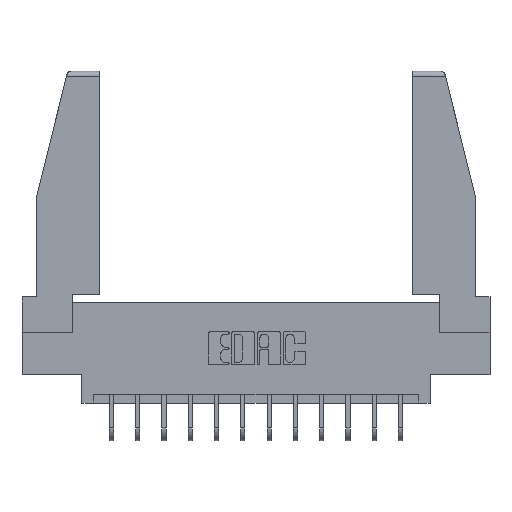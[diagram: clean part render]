
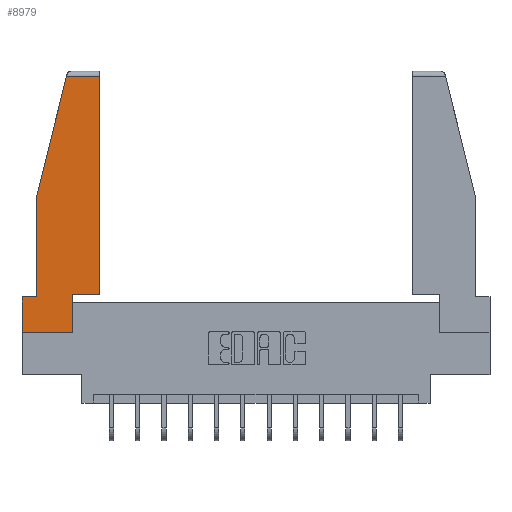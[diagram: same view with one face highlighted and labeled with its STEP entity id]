
A CAD part, top view. The second image highlights one B-rep face of the part: STEP entity #8979.
In plain terms, the highlighted planar face has unit normal (0, 0, 1).
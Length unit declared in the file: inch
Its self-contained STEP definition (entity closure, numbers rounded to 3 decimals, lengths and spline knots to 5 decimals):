
#49 = EDGE_CURVE ( 'NONE', #13625, #11015, #2145, .T. ) ;
#232 = VERTEX_POINT ( 'NONE', #2758 ) ;
#408 = VECTOR ( 'NONE', #13211, 39.37008 ) ;
#490 = EDGE_CURVE ( 'NONE', #7748, #13591, #14884, .T. ) ;
#897 = EDGE_CURVE ( 'NONE', #13152, #232, #10774, .T. ) ;
#978 = CARTESIAN_POINT ( 'NONE',  ( 0.2636, 1.52, 0. ) ) ;
#984 = ORIENTED_EDGE ( 'NONE', *, *, #7781, .T. ) ;
#1458 = VECTOR ( 'NONE', #5502, 39.37008 ) ;
#1539 = VERTEX_POINT ( 'NONE', #7104 ) ;
#1576 = VECTOR ( 'NONE', #16699, 39.37008 ) ;
#1674 = CARTESIAN_POINT ( 'NONE',  ( 0.461, 0.223, 0. ) ) ;
#1942 = EDGE_LOOP ( 'NONE', ( #7460, #984, #12631, #12615, #10129, #14130, #6817, #7483, #10998 ) ) ;
#2145 = LINE ( 'NONE', #3732, #12756 ) ;
#2707 = LINE ( 'NONE', #12174, #9495 ) ;
#2758 = CARTESIAN_POINT ( 'NONE',  ( 0.461, 1.52, 0. ) ) ;
#2829 = LINE ( 'NONE', #11694, #17472 ) ;
#3081 = DIRECTION ( 'NONE',  ( -1., 0., 0. ) ) ;
#3732 = CARTESIAN_POINT ( 'NONE',  ( 0.271, 1.55, 0. ) ) ;
#3758 = CARTESIAN_POINT ( 'NONE',  ( 0.297, 0., 0. ) ) ;
#4206 = CARTESIAN_POINT ( 'NONE',  ( 0., 1.52, 0. ) ) ;
#4217 = DIRECTION ( 'NONE',  ( 1., 0., 0. ) ) ;
#4282 = LINE ( 'NONE', #12461, #16046 ) ;
#4721 = LINE ( 'NONE', #16813, #1576 ) ;
#4820 = VECTOR ( 'NONE', #13978, 39.37008 ) ;
#4867 = LINE ( 'NONE', #9330, #8930 ) ;
#5502 = DIRECTION ( 'NONE',  ( -1., 0., 0. ) ) ;
#5700 = CARTESIAN_POINT ( 'NONE',  ( 0., 0., 0. ) ) ;
#5884 = CARTESIAN_POINT ( 'NONE',  ( 0.297, 0.223, 0. ) ) ;
#6040 = VERTEX_POINT ( 'NONE', #8866 ) ;
#6221 = VERTEX_POINT ( 'NONE', #7321 ) ;
#6622 = DIRECTION ( 'NONE',  ( 0., -1., 0. ) ) ;
#6817 = ORIENTED_EDGE ( 'NONE', *, *, #13271, .T. ) ;
#6979 = DIRECTION ( 'NONE',  ( 0., 0., 1. ) ) ;
#7104 = CARTESIAN_POINT ( 'NONE',  ( 0.086, 0.21, 0. ) ) ;
#7321 = CARTESIAN_POINT ( 'NONE',  ( 0., 0., 0. ) ) ;
#7460 = ORIENTED_EDGE ( 'NONE', *, *, #897, .T. ) ;
#7483 = ORIENTED_EDGE ( 'NONE', *, *, #490, .T. ) ;
#7748 = VERTEX_POINT ( 'NONE', #16671 ) ;
#7781 = EDGE_CURVE ( 'NONE', #232, #13625, #12934, .T. ) ;
#8866 = CARTESIAN_POINT ( 'NONE',  ( 0., 0.21, 0. ) ) ;
#8930 = VECTOR ( 'NONE', #3081, 39.37008 ) ;
#8979 = ADVANCED_FACE ( 'NONE', ( #10096 ), #15154, .T. ) ;
#9330 = CARTESIAN_POINT ( 'NONE',  ( 0., 0.21, 0. ) ) ;
#9495 = VECTOR ( 'NONE', #6622, 39.37008 ) ;
#9654 = DIRECTION ( 'NONE',  ( 0., -1., 0. ) ) ;
#10096 = FACE_OUTER_BOUND ( 'NONE', #1942, .T. ) ;
#10129 = ORIENTED_EDGE ( 'NONE', *, *, #14770, .T. ) ;
#10391 = EDGE_CURVE ( 'NONE', #6040, #6221, #4282, .T. ) ;
#10774 = LINE ( 'NONE', #12775, #4820 ) ;
#10998 = ORIENTED_EDGE ( 'NONE', *, *, #13348, .T. ) ;
#11015 = VERTEX_POINT ( 'NONE', #15110 ) ;
#11651 = EDGE_CURVE ( 'NONE', #11015, #1539, #2707, .T. ) ;
#11694 = CARTESIAN_POINT ( 'NONE',  ( 0., 0., 0. ) ) ;
#12174 = CARTESIAN_POINT ( 'NONE',  ( 0.086, 0.8, 0. ) ) ;
#12356 = AXIS2_PLACEMENT_3D ( 'NONE', #5700, #6979, #4217 ) ;
#12461 = CARTESIAN_POINT ( 'NONE',  ( 0., 0.21, 0. ) ) ;
#12615 = ORIENTED_EDGE ( 'NONE', *, *, #11651, .T. ) ;
#12631 = ORIENTED_EDGE ( 'NONE', *, *, #49, .T. ) ;
#12756 = VECTOR ( 'NONE', #17279, 39.37008 ) ;
#12775 = CARTESIAN_POINT ( 'NONE',  ( 0.461, 0.223, 0. ) ) ;
#12934 = LINE ( 'NONE', #4206, #1458 ) ;
#13152 = VERTEX_POINT ( 'NONE', #1674 ) ;
#13211 = DIRECTION ( 'NONE',  ( 0., 1., 0. ) ) ;
#13271 = EDGE_CURVE ( 'NONE', #6221, #7748, #2829, .T. ) ;
#13348 = EDGE_CURVE ( 'NONE', #13591, #13152, #4721, .T. ) ;
#13591 = VERTEX_POINT ( 'NONE', #5884 ) ;
#13625 = VERTEX_POINT ( 'NONE', #978 ) ;
#13978 = DIRECTION ( 'NONE',  ( 0., 1., 0. ) ) ;
#14130 = ORIENTED_EDGE ( 'NONE', *, *, #10391, .T. ) ;
#14770 = EDGE_CURVE ( 'NONE', #1539, #6040, #4867, .T. ) ;
#14884 = LINE ( 'NONE', #3758, #408 ) ;
#15110 = CARTESIAN_POINT ( 'NONE',  ( 0.086, 0.8, 0. ) ) ;
#15154 = PLANE ( 'NONE',  #12356 ) ;
#15358 = DIRECTION ( 'NONE',  ( 1., 0., 0. ) ) ;
#16046 = VECTOR ( 'NONE', #9654, 39.37008 ) ;
#16671 = CARTESIAN_POINT ( 'NONE',  ( 0.297, 0., 0. ) ) ;
#16699 = DIRECTION ( 'NONE',  ( 1., 0., 0. ) ) ;
#16813 = CARTESIAN_POINT ( 'NONE',  ( 0.297, 0.223, 0. ) ) ;
#17279 = DIRECTION ( 'NONE',  ( -0.239, -0.971, 0. ) ) ;
#17472 = VECTOR ( 'NONE', #15358, 39.37008 ) ;
